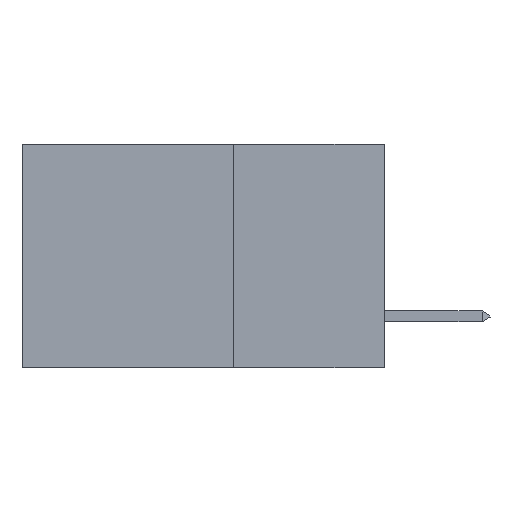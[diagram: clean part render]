
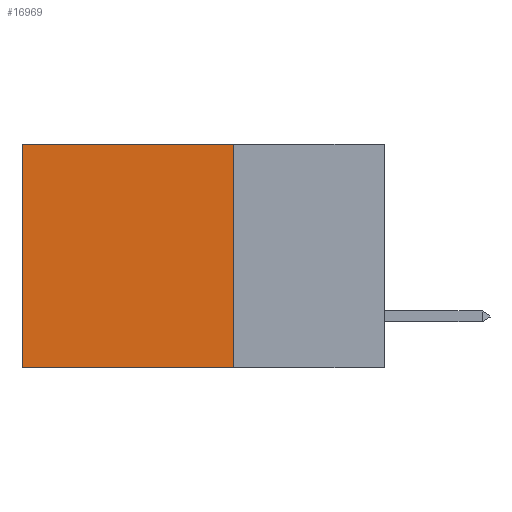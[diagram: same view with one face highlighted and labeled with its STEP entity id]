
A CAD part, left-side view. The second image highlights one B-rep face of the part: STEP entity #16969.
In plain terms, the highlighted planar face has unit normal (-1, 0, 0).
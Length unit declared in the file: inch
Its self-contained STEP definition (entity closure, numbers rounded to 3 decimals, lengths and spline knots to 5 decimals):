
#1972 = EDGE_CURVE ( 'NONE', #15116, #15798, #3118, .T. ) ;
#2166 = VECTOR ( 'NONE', #19087, 39.37008 ) ;
#2257 = CARTESIAN_POINT ( 'NONE',  ( 0.2875, 0.25, -0.37 ) ) ;
#2506 = PLANE ( 'NONE',  #17013 ) ;
#2533 = CARTESIAN_POINT ( 'NONE',  ( 0.2875, 0.6, 0. ) ) ;
#2897 = DIRECTION ( 'NONE',  ( 0., 1., 0. ) ) ;
#3118 = LINE ( 'NONE', #15478, #13901 ) ;
#3451 = LINE ( 'NONE', #2533, #2166 ) ;
#3490 = FACE_OUTER_BOUND ( 'NONE', #6079, .T. ) ;
#3585 = CARTESIAN_POINT ( 'NONE',  ( 0.2875, 0.25, 0. ) ) ;
#3880 = CARTESIAN_POINT ( 'NONE',  ( 0.2875, 0.6, 0. ) ) ;
#4172 = VECTOR ( 'NONE', #2897, 39.37008 ) ;
#4224 = DIRECTION ( 'NONE',  ( 1., 0., 0. ) ) ;
#5392 = CARTESIAN_POINT ( 'NONE',  ( 0.2875, 0.25, 0. ) ) ;
#6079 = EDGE_LOOP ( 'NONE', ( #7015, #14020, #13917, #11197 ) ) ;
#6652 = DIRECTION ( 'NONE',  ( 0., 0., -1. ) ) ;
#7015 = ORIENTED_EDGE ( 'NONE', *, *, #7470, .T. ) ;
#7470 = EDGE_CURVE ( 'NONE', #15798, #20987, #3451, .T. ) ;
#7516 = EDGE_CURVE ( 'NONE', #15116, #12069, #20381, .T. ) ;
#8553 = LINE ( 'NONE', #15816, #4172 ) ;
#9087 = DIRECTION ( 'NONE',  ( 0., 1., 0. ) ) ;
#10601 = DIRECTION ( 'NONE',  ( 0., 0., -1. ) ) ;
#11119 = VECTOR ( 'NONE', #6652, 39.37008 ) ;
#11197 = ORIENTED_EDGE ( 'NONE', *, *, #1972, .T. ) ;
#12069 = VERTEX_POINT ( 'NONE', #2257 ) ;
#12332 = EDGE_CURVE ( 'NONE', #12069, #20987, #8553, .T. ) ;
#13901 = VECTOR ( 'NONE', #9087, 39.37008 ) ;
#13917 = ORIENTED_EDGE ( 'NONE', *, *, #7516, .F. ) ;
#14020 = ORIENTED_EDGE ( 'NONE', *, *, #12332, .F. ) ;
#15116 = VERTEX_POINT ( 'NONE', #5392 ) ;
#15478 = CARTESIAN_POINT ( 'NONE',  ( 0.2875, 0.25, 0. ) ) ;
#15798 = VERTEX_POINT ( 'NONE', #3880 ) ;
#15816 = CARTESIAN_POINT ( 'NONE',  ( 0.2875, 0.25, -0.37 ) ) ;
#16969 = ADVANCED_FACE ( 'NONE', ( #3490 ), #2506, .F. ) ;
#17013 = AXIS2_PLACEMENT_3D ( 'NONE', #20443, #4224, #10601 ) ;
#19087 = DIRECTION ( 'NONE',  ( 0., 0., -1. ) ) ;
#20381 = LINE ( 'NONE', #3585, #11119 ) ;
#20443 = CARTESIAN_POINT ( 'NONE',  ( 0.2875, 0.25, 0. ) ) ;
#20577 = CARTESIAN_POINT ( 'NONE',  ( 0.2875, 0.6, -0.37 ) ) ;
#20987 = VERTEX_POINT ( 'NONE', #20577 ) ;
